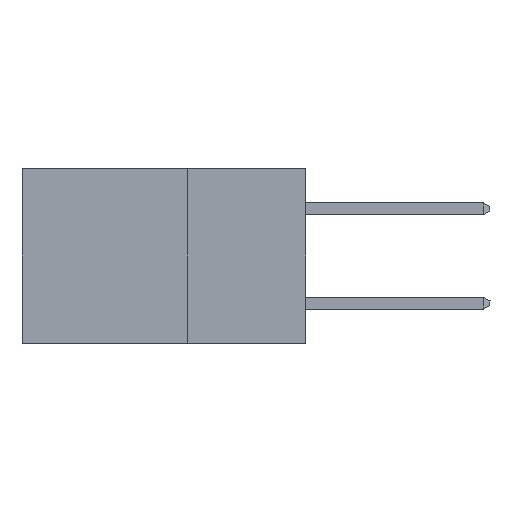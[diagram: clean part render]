
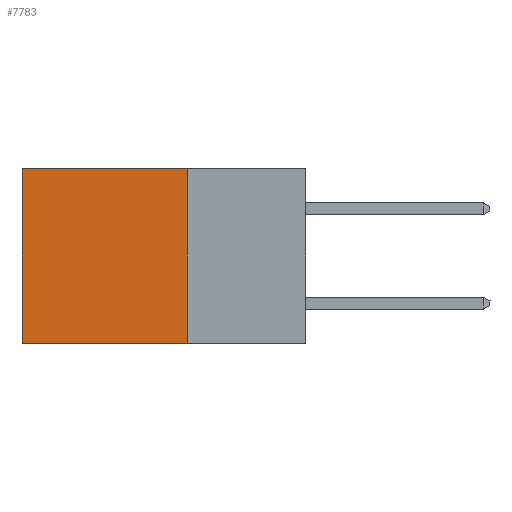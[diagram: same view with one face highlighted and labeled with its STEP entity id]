
A CAD part, left-side view. The second image highlights one B-rep face of the part: STEP entity #7783.
In plain terms, the highlighted planar face has unit normal (-1, 0, 0).
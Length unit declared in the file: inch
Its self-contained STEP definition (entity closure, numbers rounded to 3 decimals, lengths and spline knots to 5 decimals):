
#47 = CARTESIAN_POINT ( 'NONE',  ( 0.298, 0.25, 0. ) ) ;
#539 = VECTOR ( 'NONE', #6579, 39.37008 ) ;
#692 = DIRECTION ( 'NONE',  ( 0., 1., 0. ) ) ;
#1195 = VERTEX_POINT ( 'NONE', #6967 ) ;
#1621 = EDGE_CURVE ( 'NONE', #8512, #6002, #8356, .T. ) ;
#1729 = CARTESIAN_POINT ( 'NONE',  ( 0.298, 0.6, 0. ) ) ;
#2282 = LINE ( 'NONE', #47, #6420 ) ;
#2379 = CARTESIAN_POINT ( 'NONE',  ( 0.298, 0.25, -0.37 ) ) ;
#2658 = FACE_OUTER_BOUND ( 'NONE', #6745, .T. ) ;
#2793 = ORIENTED_EDGE ( 'NONE', *, *, #4085, .T. ) ;
#2987 = LINE ( 'NONE', #10614, #539 ) ;
#3076 = CARTESIAN_POINT ( 'NONE',  ( 0.298, 0.25, -0.37 ) ) ;
#3737 = PLANE ( 'NONE',  #8221 ) ;
#4085 = EDGE_CURVE ( 'NONE', #10183, #6002, #5886, .T. ) ;
#4446 = VECTOR ( 'NONE', #7008, 39.37008 ) ;
#4992 = ORIENTED_EDGE ( 'NONE', *, *, #1621, .F. ) ;
#5354 = DIRECTION ( 'NONE',  ( 0., 0., -1. ) ) ;
#5886 = LINE ( 'NONE', #7043, #4446 ) ;
#6002 = VERTEX_POINT ( 'NONE', #7695 ) ;
#6420 = VECTOR ( 'NONE', #7517, 39.37008 ) ;
#6579 = DIRECTION ( 'NONE',  ( 0., 1., 0. ) ) ;
#6745 = EDGE_LOOP ( 'NONE', ( #2793, #4992, #9687, #7497 ) ) ;
#6966 = DIRECTION ( 'NONE',  ( 1., 0., 0. ) ) ;
#6967 = CARTESIAN_POINT ( 'NONE',  ( 0.298, 0.25, 0. ) ) ;
#7008 = DIRECTION ( 'NONE',  ( 0., 0., -1. ) ) ;
#7043 = CARTESIAN_POINT ( 'NONE',  ( 0.298, 0.6, 0. ) ) ;
#7497 = ORIENTED_EDGE ( 'NONE', *, *, #10569, .T. ) ;
#7517 = DIRECTION ( 'NONE',  ( 0., 0., -1. ) ) ;
#7596 = EDGE_CURVE ( 'NONE', #1195, #8512, #2282, .T. ) ;
#7695 = CARTESIAN_POINT ( 'NONE',  ( 0.298, 0.6, -0.37 ) ) ;
#7783 = ADVANCED_FACE ( 'NONE', ( #2658 ), #3737, .F. ) ;
#7967 = VECTOR ( 'NONE', #692, 39.37008 ) ;
#8221 = AXIS2_PLACEMENT_3D ( 'NONE', #9456, #6966, #5354 ) ;
#8356 = LINE ( 'NONE', #3076, #7967 ) ;
#8512 = VERTEX_POINT ( 'NONE', #2379 ) ;
#9456 = CARTESIAN_POINT ( 'NONE',  ( 0.298, 0.25, 0. ) ) ;
#9687 = ORIENTED_EDGE ( 'NONE', *, *, #7596, .F. ) ;
#10183 = VERTEX_POINT ( 'NONE', #1729 ) ;
#10569 = EDGE_CURVE ( 'NONE', #1195, #10183, #2987, .T. ) ;
#10614 = CARTESIAN_POINT ( 'NONE',  ( 0.298, 0.25, 0. ) ) ;
